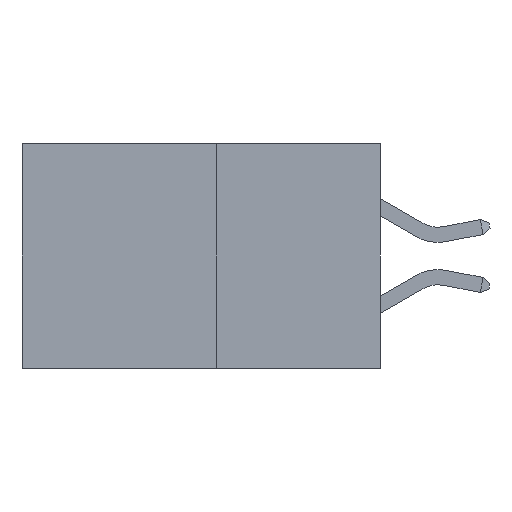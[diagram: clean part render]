
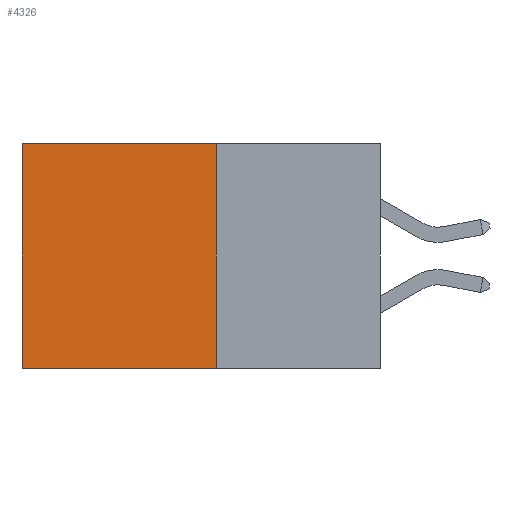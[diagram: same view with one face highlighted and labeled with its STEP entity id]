
A CAD part, left-side view. The second image highlights one B-rep face of the part: STEP entity #4326.
In plain terms, the highlighted planar face has unit normal (-1, 0, 0).
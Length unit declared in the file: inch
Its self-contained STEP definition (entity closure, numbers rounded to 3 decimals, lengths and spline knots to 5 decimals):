
#2 = VERTEX_POINT ( 'NONE', #9485 ) ;
#217 = CARTESIAN_POINT ( 'NONE',  ( 0.277, 0.27, 0. ) ) ;
#388 = CARTESIAN_POINT ( 'NONE',  ( 0.277, 0.59, 0. ) ) ;
#545 = EDGE_CURVE ( 'NONE', #2, #9849, #7431, .T. ) ;
#1246 = VECTOR ( 'NONE', #3010, 39.37008 ) ;
#1479 = LINE ( 'NONE', #8333, #6002 ) ;
#1571 = ORIENTED_EDGE ( 'NONE', *, *, #1710, .T. ) ;
#1663 = ORIENTED_EDGE ( 'NONE', *, *, #3909, .F. ) ;
#1704 = ORIENTED_EDGE ( 'NONE', *, *, #2097, .F. ) ;
#1710 = EDGE_CURVE ( 'NONE', #9849, #8368, #9716, .T. ) ;
#1735 = ORIENTED_EDGE ( 'NONE', *, *, #545, .T. ) ;
#1845 = FACE_OUTER_BOUND ( 'NONE', #2742, .T. ) ;
#2097 = EDGE_CURVE ( 'NONE', #2, #8300, #8122, .T. ) ;
#2302 = DIRECTION ( 'NONE',  ( 0., 1., 0. ) ) ;
#2742 = EDGE_LOOP ( 'NONE', ( #1571, #1663, #1704, #1735 ) ) ;
#3010 = DIRECTION ( 'NONE',  ( 0., 0., -1. ) ) ;
#3909 = EDGE_CURVE ( 'NONE', #8300, #8368, #1479, .T. ) ;
#4326 = ADVANCED_FACE ( 'NONE', ( #1845 ), #5458, .F. ) ;
#5430 = VECTOR ( 'NONE', #7506, 39.37008 ) ;
#5458 = PLANE ( 'NONE',  #8444 ) ;
#5743 = VECTOR ( 'NONE', #10218, 39.37008 ) ;
#6002 = VECTOR ( 'NONE', #2302, 39.37008 ) ;
#7318 = CARTESIAN_POINT ( 'NONE',  ( 0.277, 0.27, -0.37 ) ) ;
#7339 = CARTESIAN_POINT ( 'NONE',  ( 0.277, 0.59, -0.37 ) ) ;
#7431 = LINE ( 'NONE', #217, #5430 ) ;
#7506 = DIRECTION ( 'NONE',  ( 0., 1., 0. ) ) ;
#7854 = DIRECTION ( 'NONE',  ( 1., 0., 0. ) ) ;
#8122 = LINE ( 'NONE', #10661, #1246 ) ;
#8300 = VERTEX_POINT ( 'NONE', #9980 ) ;
#8333 = CARTESIAN_POINT ( 'NONE',  ( 0.277, 0.27, -0.37 ) ) ;
#8368 = VERTEX_POINT ( 'NONE', #10532 ) ;
#8444 = AXIS2_PLACEMENT_3D ( 'NONE', #7318, #7854, #9042 ) ;
#9042 = DIRECTION ( 'NONE',  ( 0., 0., -1. ) ) ;
#9485 = CARTESIAN_POINT ( 'NONE',  ( 0.277, 0.27, 0. ) ) ;
#9716 = LINE ( 'NONE', #7339, #5743 ) ;
#9849 = VERTEX_POINT ( 'NONE', #388 ) ;
#9980 = CARTESIAN_POINT ( 'NONE',  ( 0.277, 0.27, -0.37 ) ) ;
#10218 = DIRECTION ( 'NONE',  ( 0., 0., -1. ) ) ;
#10532 = CARTESIAN_POINT ( 'NONE',  ( 0.277, 0.59, -0.37 ) ) ;
#10661 = CARTESIAN_POINT ( 'NONE',  ( 0.277, 0.27, -0.37 ) ) ;
